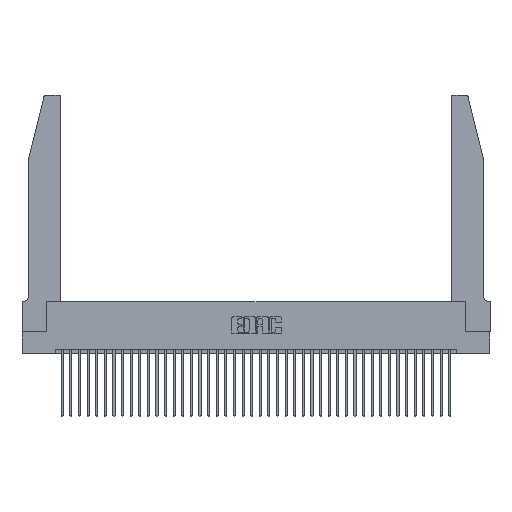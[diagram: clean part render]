
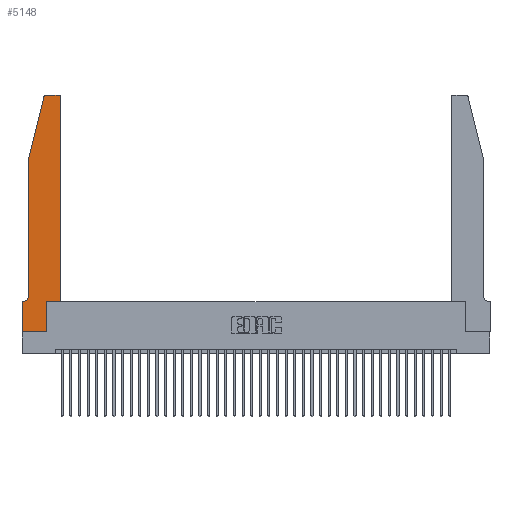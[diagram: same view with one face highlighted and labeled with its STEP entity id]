
A CAD part, top view. The second image highlights one B-rep face of the part: STEP entity #5148.
In plain terms, the highlighted planar face has unit normal (0, 0, 1).
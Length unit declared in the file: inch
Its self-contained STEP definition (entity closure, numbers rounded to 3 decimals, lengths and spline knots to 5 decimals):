
#242 = ORIENTED_EDGE ( 'NONE', *, *, #15473, .T. ) ;
#291 = CARTESIAN_POINT ( 'NONE',  ( 0.4505, 0.35, 0.37 ) ) ;
#541 = PLANE ( 'NONE',  #8002 ) ;
#684 = ORIENTED_EDGE ( 'NONE', *, *, #28292, .T. ) ;
#728 = EDGE_CURVE ( 'NONE', #2034, #38492, #11265, .T. ) ;
#1231 = CARTESIAN_POINT ( 'NONE',  ( 0.2865, 0.35, 0.37 ) ) ;
#1470 = EDGE_CURVE ( 'NONE', #31985, #9212, #18028, .T. ) ;
#1592 = DIRECTION ( 'NONE',  ( 1., 0., 0. ) ) ;
#2034 = VERTEX_POINT ( 'NONE', #5326 ) ;
#2381 = EDGE_CURVE ( 'NONE', #9233, #39079, #3167, .T. ) ;
#2404 = DIRECTION ( 'NONE',  ( 0., 0., 1. ) ) ;
#3167 = LINE ( 'NONE', #22539, #35336 ) ;
#3281 = DIRECTION ( 'NONE',  ( 0., 0., -1. ) ) ;
#3767 = DIRECTION ( 'NONE',  ( 1., 0., 0. ) ) ;
#3997 = CIRCLE ( 'NONE', #4755, 0.07 ) ;
#4755 = AXIS2_PLACEMENT_3D ( 'NONE', #22098, #3281, #25186 ) ;
#5148 = ADVANCED_FACE ( 'NONE', ( #21189 ), #541, .T. ) ;
#5324 = EDGE_CURVE ( 'NONE', #15408, #13709, #31813, .T. ) ;
#5326 = CARTESIAN_POINT ( 'NONE',  ( 0.4505, 0.35, 0.37 ) ) ;
#5425 = CARTESIAN_POINT ( 'NONE',  ( 0.4505, 0.35, 0.37 ) ) ;
#5534 = ORIENTED_EDGE ( 'NONE', *, *, #12995, .T. ) ;
#6018 = ORIENTED_EDGE ( 'NONE', *, *, #2381, .T. ) ;
#6558 = CARTESIAN_POINT ( 'NONE',  ( 0.284, 2.75, 0.37 ) ) ;
#6959 = CARTESIAN_POINT ( 'NONE',  ( 0.2865, 0.35, 0.37 ) ) ;
#7732 = VECTOR ( 'NONE', #12922, 39.37008 ) ;
#7974 = VECTOR ( 'NONE', #20111, 39.37008 ) ;
#8002 = AXIS2_PLACEMENT_3D ( 'NONE', #34829, #22557, #3767 ) ;
#8039 = ORIENTED_EDGE ( 'NONE', *, *, #5324, .T. ) ;
#9112 = ORIENTED_EDGE ( 'NONE', *, *, #37573, .T. ) ;
#9212 = VERTEX_POINT ( 'NONE', #13311 ) ;
#9233 = VERTEX_POINT ( 'NONE', #25728 ) ;
#9741 = CARTESIAN_POINT ( 'NONE',  ( 0.0055, 0.35, 0.37 ) ) ;
#9819 = ORIENTED_EDGE ( 'NONE', *, *, #13578, .T. ) ;
#10009 = DIRECTION ( 'NONE',  ( -1., 0., 0. ) ) ;
#10266 = VECTOR ( 'NONE', #27240, 39.37008 ) ;
#11265 = LINE ( 'NONE', #5425, #10266 ) ;
#12054 = DIRECTION ( 'NONE',  ( -1., 0., 0. ) ) ;
#12678 = AXIS2_PLACEMENT_3D ( 'NONE', #21234, #2404, #24349 ) ;
#12824 = VERTEX_POINT ( 'NONE', #36885 ) ;
#12922 = DIRECTION ( 'NONE',  ( -0.239, -0.971, 0. ) ) ;
#12995 = EDGE_CURVE ( 'NONE', #13709, #2034, #36844, .T. ) ;
#13311 = CARTESIAN_POINT ( 'NONE',  ( 0., 0.35, 0.37 ) ) ;
#13399 = CARTESIAN_POINT ( 'NONE',  ( 0.4505, 2.72, 0.37 ) ) ;
#13578 = EDGE_CURVE ( 'NONE', #30841, #35370, #17051, .T. ) ;
#13709 = VERTEX_POINT ( 'NONE', #6959 ) ;
#14047 = CARTESIAN_POINT ( 'NONE',  ( 0.0755, 2., 0.37 ) ) ;
#15216 = CARTESIAN_POINT ( 'NONE',  ( 0.0755, 0.35, 0.37 ) ) ;
#15408 = VERTEX_POINT ( 'NONE', #25695 ) ;
#15473 = EDGE_CURVE ( 'NONE', #9212, #12824, #15963, .T. ) ;
#15715 = DIRECTION ( 'NONE',  ( 1., 0., 0. ) ) ;
#15787 = DIRECTION ( 'NONE',  ( 0., -1., 0. ) ) ;
#15963 = LINE ( 'NONE', #29085, #32385 ) ;
#17051 = LINE ( 'NONE', #37368, #7732 ) ;
#17074 = CIRCLE ( 'NONE', #38359, 0.03 ) ;
#17427 = LINE ( 'NONE', #34254, #32909 ) ;
#17546 = EDGE_CURVE ( 'NONE', #38492, #9233, #30787, .T. ) ;
#18028 = LINE ( 'NONE', #15216, #25284 ) ;
#20111 = DIRECTION ( 'NONE',  ( 0., 1., 0. ) ) ;
#20333 = EDGE_CURVE ( 'NONE', #31246, #31985, #3997, .T. ) ;
#20456 = DIRECTION ( 'NONE',  ( 0., 0., 1. ) ) ;
#20967 = ORIENTED_EDGE ( 'NONE', *, *, #20333, .T. ) ;
#21189 = FACE_OUTER_BOUND ( 'NONE', #34050, .T. ) ;
#21234 = CARTESIAN_POINT ( 'NONE',  ( 0.4205, 2.72, 0.37 ) ) ;
#21403 = VECTOR ( 'NONE', #22315, 39.37008 ) ;
#21636 = EDGE_CURVE ( 'NONE', #12824, #15408, #39857, .T. ) ;
#21914 = ORIENTED_EDGE ( 'NONE', *, *, #728, .T. ) ;
#22098 = CARTESIAN_POINT ( 'NONE',  ( 0.0055, 0.42, 0.37 ) ) ;
#22315 = DIRECTION ( 'NONE',  ( 1., 0., 0. ) ) ;
#22526 = VECTOR ( 'NONE', #15715, 39.37008 ) ;
#22539 = CARTESIAN_POINT ( 'NONE',  ( 0.2605, 2.75, 0.37 ) ) ;
#22557 = DIRECTION ( 'NONE',  ( 0., 0., 1. ) ) ;
#24349 = DIRECTION ( 'NONE',  ( 1., 0., 0. ) ) ;
#25186 = DIRECTION ( 'NONE',  ( -1., 0., 0. ) ) ;
#25193 = CARTESIAN_POINT ( 'NONE',  ( 0.25487, 2.72718, 0.37 ) ) ;
#25284 = VECTOR ( 'NONE', #12054, 39.37008 ) ;
#25695 = CARTESIAN_POINT ( 'NONE',  ( 0.2865, 0., 0.37 ) ) ;
#25728 = CARTESIAN_POINT ( 'NONE',  ( 0.4205, 2.75, 0.37 ) ) ;
#27057 = CARTESIAN_POINT ( 'NONE',  ( 0.0755, 0.42, 0.37 ) ) ;
#27240 = DIRECTION ( 'NONE',  ( 0., 1., 0. ) ) ;
#28292 = EDGE_CURVE ( 'NONE', #35370, #31246, #17427, .T. ) ;
#29085 = CARTESIAN_POINT ( 'NONE',  ( 0., 0., 0.37 ) ) ;
#30092 = ORIENTED_EDGE ( 'NONE', *, *, #1470, .T. ) ;
#30281 = ORIENTED_EDGE ( 'NONE', *, *, #21636, .T. ) ;
#30787 = CIRCLE ( 'NONE', #12678, 0.03 ) ;
#30841 = VERTEX_POINT ( 'NONE', #25193 ) ;
#31246 = VERTEX_POINT ( 'NONE', #27057 ) ;
#31813 = LINE ( 'NONE', #1231, #7974 ) ;
#31985 = VERTEX_POINT ( 'NONE', #9741 ) ;
#32200 = DIRECTION ( 'NONE',  ( 0., -1., 0. ) ) ;
#32385 = VECTOR ( 'NONE', #32200, 39.37008 ) ;
#32909 = VECTOR ( 'NONE', #15787, 39.37008 ) ;
#34050 = EDGE_LOOP ( 'NONE', ( #6018, #9112, #9819, #684, #20967, #30092, #242, #30281, #8039, #5534, #21914, #38819 ) ) ;
#34254 = CARTESIAN_POINT ( 'NONE',  ( 0.0755, 2., 0.37 ) ) ;
#34829 = CARTESIAN_POINT ( 'NONE',  ( 0., 0.35, 0.37 ) ) ;
#35336 = VECTOR ( 'NONE', #10009, 39.37008 ) ;
#35370 = VERTEX_POINT ( 'NONE', #14047 ) ;
#36844 = LINE ( 'NONE', #291, #21403 ) ;
#36885 = CARTESIAN_POINT ( 'NONE',  ( 0., 0., 0.37 ) ) ;
#37259 = CARTESIAN_POINT ( 'NONE',  ( 0., 0., 0.37 ) ) ;
#37368 = CARTESIAN_POINT ( 'NONE',  ( 0.0755, 2., 0.37 ) ) ;
#37573 = EDGE_CURVE ( 'NONE', #39079, #30841, #17074, .T. ) ;
#38359 = AXIS2_PLACEMENT_3D ( 'NONE', #38905, #20456, #1592 ) ;
#38492 = VERTEX_POINT ( 'NONE', #13399 ) ;
#38819 = ORIENTED_EDGE ( 'NONE', *, *, #17546, .T. ) ;
#38905 = CARTESIAN_POINT ( 'NONE',  ( 0.284, 2.72, 0.37 ) ) ;
#39079 = VERTEX_POINT ( 'NONE', #6558 ) ;
#39857 = LINE ( 'NONE', #37259, #22526 ) ;
